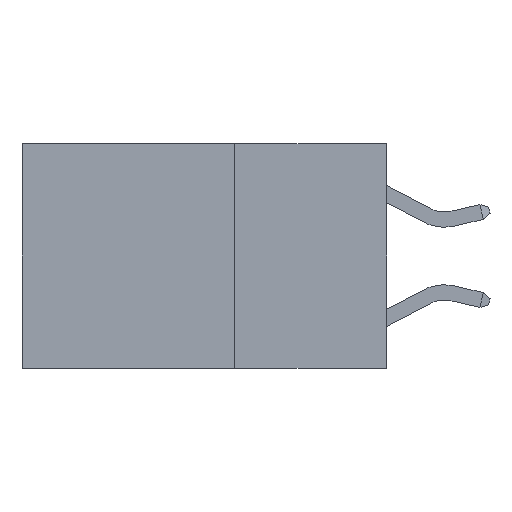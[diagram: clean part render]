
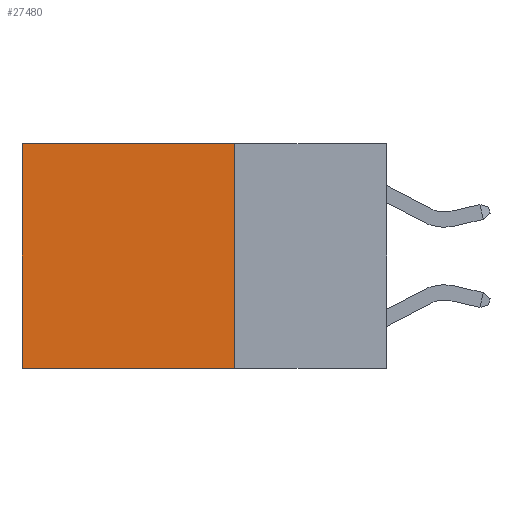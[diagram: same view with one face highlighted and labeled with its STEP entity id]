
A CAD part, left-side view. The second image highlights one B-rep face of the part: STEP entity #27480.
In plain terms, the highlighted planar face has unit normal (-1, 0, 0).
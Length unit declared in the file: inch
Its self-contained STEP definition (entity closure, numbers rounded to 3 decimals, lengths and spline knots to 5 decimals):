
#323 = CARTESIAN_POINT ( 'NONE',  ( 0.2625, 0.25, -0.37 ) ) ;
#368 = DIRECTION ( 'NONE',  ( 0., 0., -1. ) ) ;
#590 = EDGE_LOOP ( 'NONE', ( #26693, #27444, #13295, #10916 ) ) ;
#713 = VERTEX_POINT ( 'NONE', #11117 ) ;
#1212 = CARTESIAN_POINT ( 'NONE',  ( 0.2625, 0.25, 0. ) ) ;
#1499 = CARTESIAN_POINT ( 'NONE',  ( 0.2625, 0.6, 0. ) ) ;
#2345 = PLANE ( 'NONE',  #22716 ) ;
#2840 = EDGE_CURVE ( 'NONE', #713, #18747, #25194, .T. ) ;
#4563 = FACE_OUTER_BOUND ( 'NONE', #590, .T. ) ;
#5790 = LINE ( 'NONE', #1499, #13699 ) ;
#7050 = VERTEX_POINT ( 'NONE', #323 ) ;
#7060 = CARTESIAN_POINT ( 'NONE',  ( 0.2625, 0.25, 0. ) ) ;
#8106 = CARTESIAN_POINT ( 'NONE',  ( 0.2625, 0.6, -0.37 ) ) ;
#9376 = LINE ( 'NONE', #1212, #25615 ) ;
#10916 = ORIENTED_EDGE ( 'NONE', *, *, #2840, .T. ) ;
#11117 = CARTESIAN_POINT ( 'NONE',  ( 0.2625, 0.25, 0. ) ) ;
#11420 = LINE ( 'NONE', #13188, #16310 ) ;
#12866 = VERTEX_POINT ( 'NONE', #8106 ) ;
#13188 = CARTESIAN_POINT ( 'NONE',  ( 0.2625, 0.25, -0.37 ) ) ;
#13295 = ORIENTED_EDGE ( 'NONE', *, *, #28414, .F. ) ;
#13699 = VECTOR ( 'NONE', #28335, 39.37008 ) ;
#16310 = VECTOR ( 'NONE', #17772, 39.37008 ) ;
#17772 = DIRECTION ( 'NONE',  ( 0., 1., 0. ) ) ;
#18747 = VERTEX_POINT ( 'NONE', #20118 ) ;
#20118 = CARTESIAN_POINT ( 'NONE',  ( 0.2625, 0.6, 0. ) ) ;
#20270 = DIRECTION ( 'NONE',  ( 1., 0., 0. ) ) ;
#22645 = DIRECTION ( 'NONE',  ( 0., 0., -1. ) ) ;
#22716 = AXIS2_PLACEMENT_3D ( 'NONE', #7060, #20270, #22645 ) ;
#23515 = EDGE_CURVE ( 'NONE', #7050, #12866, #11420, .T. ) ;
#24036 = EDGE_CURVE ( 'NONE', #18747, #12866, #5790, .T. ) ;
#25194 = LINE ( 'NONE', #25478, #28697 ) ;
#25478 = CARTESIAN_POINT ( 'NONE',  ( 0.2625, 0.25, 0. ) ) ;
#25615 = VECTOR ( 'NONE', #368, 39.37008 ) ;
#26693 = ORIENTED_EDGE ( 'NONE', *, *, #24036, .T. ) ;
#27444 = ORIENTED_EDGE ( 'NONE', *, *, #23515, .F. ) ;
#27480 = ADVANCED_FACE ( 'NONE', ( #4563 ), #2345, .F. ) ;
#27561 = DIRECTION ( 'NONE',  ( 0., 1., 0. ) ) ;
#28335 = DIRECTION ( 'NONE',  ( 0., 0., -1. ) ) ;
#28414 = EDGE_CURVE ( 'NONE', #713, #7050, #9376, .T. ) ;
#28697 = VECTOR ( 'NONE', #27561, 39.37008 ) ;
